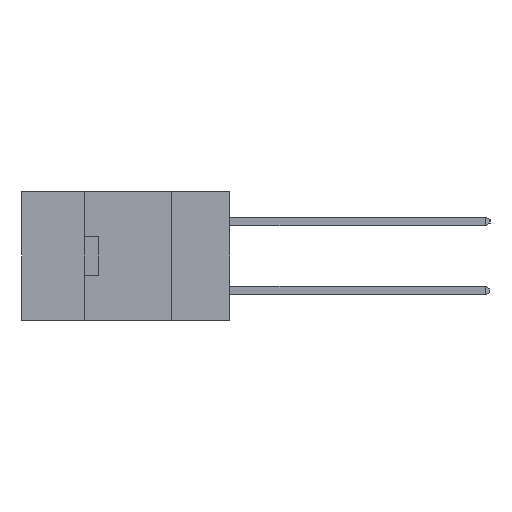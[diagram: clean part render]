
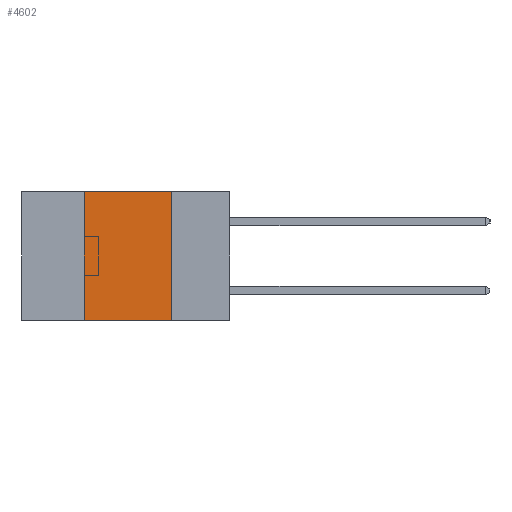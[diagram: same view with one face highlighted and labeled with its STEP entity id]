
A CAD part, left-side view. The second image highlights one B-rep face of the part: STEP entity #4602.
In plain terms, the highlighted planar face has unit normal (-1, 0, 0).
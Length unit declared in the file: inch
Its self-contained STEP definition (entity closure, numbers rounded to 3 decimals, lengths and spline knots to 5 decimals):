
#4 = ORIENTED_EDGE ( 'NONE', *, *, #16210, .F. ) ;
#710 = CARTESIAN_POINT ( 'NONE',  ( 0., 0.6, 0. ) ) ;
#2995 = DIRECTION ( 'NONE',  ( 0., 0., -1. ) ) ;
#4283 = CARTESIAN_POINT ( 'NONE',  ( 0., 0.17, 0. ) ) ;
#4602 = ADVANCED_FACE ( 'NONE', ( #28040 ), #22517, .F. ) ;
#6152 = EDGE_CURVE ( 'NONE', #13350, #24979, #9945, .T. ) ;
#6749 = CARTESIAN_POINT ( 'NONE',  ( 0., 0.6, 0. ) ) ;
#8648 = VECTOR ( 'NONE', #17601, 39.37008 ) ;
#9344 = LINE ( 'NONE', #6749, #8648 ) ;
#9945 = LINE ( 'NONE', #27390, #20116 ) ;
#10003 = LINE ( 'NONE', #13907, #15791 ) ;
#10359 = VERTEX_POINT ( 'NONE', #4283 ) ;
#11316 = EDGE_CURVE ( 'NONE', #13350, #18660, #10003, .T. ) ;
#11471 = CARTESIAN_POINT ( 'NONE',  ( 0., 0.17, -0.37 ) ) ;
#12017 = VECTOR ( 'NONE', #15741, 39.37008 ) ;
#12704 = LINE ( 'NONE', #11471, #12017 ) ;
#13350 = VERTEX_POINT ( 'NONE', #13634 ) ;
#13634 = CARTESIAN_POINT ( 'NONE',  ( 0., 0.42, -0.37 ) ) ;
#13907 = CARTESIAN_POINT ( 'NONE',  ( 0., 0.6, -0.37 ) ) ;
#15226 = AXIS2_PLACEMENT_3D ( 'NONE', #710, #16108, #2995 ) ;
#15741 = DIRECTION ( 'NONE',  ( 0., 0., -1. ) ) ;
#15791 = VECTOR ( 'NONE', #16078, 39.37008 ) ;
#16078 = DIRECTION ( 'NONE',  ( 0., -1., 0. ) ) ;
#16108 = DIRECTION ( 'NONE',  ( 1., 0., 0. ) ) ;
#16210 = EDGE_CURVE ( 'NONE', #24979, #10359, #9344, .T. ) ;
#16522 = ORIENTED_EDGE ( 'NONE', *, *, #6152, .F. ) ;
#17601 = DIRECTION ( 'NONE',  ( 0., -1., 0. ) ) ;
#18583 = ORIENTED_EDGE ( 'NONE', *, *, #20540, .F. ) ;
#18660 = VERTEX_POINT ( 'NONE', #27883 ) ;
#18866 = DIRECTION ( 'NONE',  ( 0., 0., 1. ) ) ;
#20116 = VECTOR ( 'NONE', #18866, 39.37008 ) ;
#20540 = EDGE_CURVE ( 'NONE', #10359, #18660, #12704, .T. ) ;
#22517 = PLANE ( 'NONE',  #15226 ) ;
#24979 = VERTEX_POINT ( 'NONE', #27062 ) ;
#25991 = EDGE_LOOP ( 'NONE', ( #18583, #4, #16522, #26974 ) ) ;
#26974 = ORIENTED_EDGE ( 'NONE', *, *, #11316, .T. ) ;
#27062 = CARTESIAN_POINT ( 'NONE',  ( 0., 0.42, 0. ) ) ;
#27390 = CARTESIAN_POINT ( 'NONE',  ( 0., 0.42, -0.37 ) ) ;
#27883 = CARTESIAN_POINT ( 'NONE',  ( 0., 0.17, -0.37 ) ) ;
#28040 = FACE_OUTER_BOUND ( 'NONE', #25991, .T. ) ;
